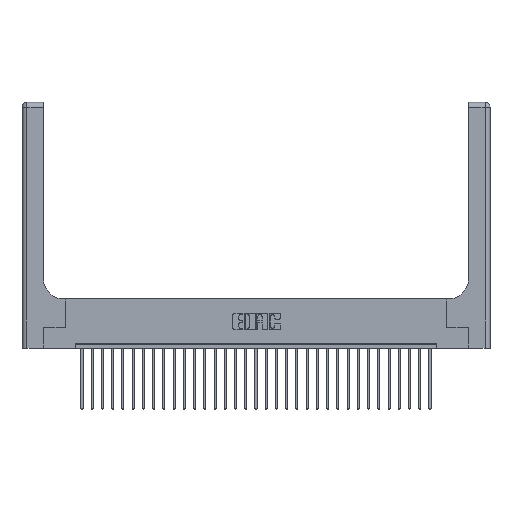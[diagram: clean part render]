
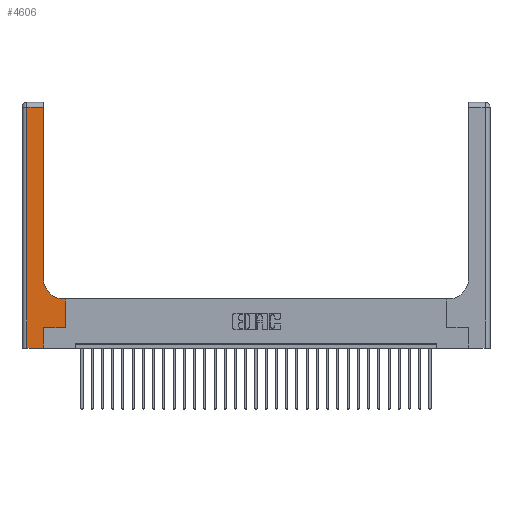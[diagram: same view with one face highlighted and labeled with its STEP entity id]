
A CAD part, top view. The second image highlights one B-rep face of the part: STEP entity #4606.
In plain terms, the highlighted planar face has unit normal (0, 0, 1).
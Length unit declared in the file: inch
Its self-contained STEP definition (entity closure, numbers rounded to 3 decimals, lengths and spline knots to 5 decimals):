
#72 = CARTESIAN_POINT ( 'NONE',  ( 0.26, 3., 0.37 ) ) ;
#588 = CARTESIAN_POINT ( 'NONE',  ( 0.265, 0.25, 0.37 ) ) ;
#1229 = CARTESIAN_POINT ( 'NONE',  ( 0., 0., 0.37 ) ) ;
#1297 = VECTOR ( 'NONE', #9552, 39.37008 ) ;
#1741 = LINE ( 'NONE', #25455, #25307 ) ;
#2475 = EDGE_CURVE ( 'NONE', #23902, #25149, #2634, .T. ) ;
#2634 = LINE ( 'NONE', #17850, #22500 ) ;
#3107 = CARTESIAN_POINT ( 'NONE',  ( 0.26, 2.94, 0.37 ) ) ;
#3252 = VERTEX_POINT ( 'NONE', #21655 ) ;
#3727 = AXIS2_PLACEMENT_3D ( 'NONE', #21616, #21528, #19169 ) ;
#3817 = CIRCLE ( 'NONE', #18134, 0.25 ) ;
#4252 = PLANE ( 'NONE',  #3727 ) ;
#4606 = ADVANCED_FACE ( 'NONE', ( #6534 ), #4252, .F. ) ;
#5567 = DIRECTION ( 'NONE',  ( 0., 0., -1. ) ) ;
#6486 = LINE ( 'NONE', #17492, #7158 ) ;
#6534 = FACE_OUTER_BOUND ( 'NONE', #21782, .T. ) ;
#6974 = LINE ( 'NONE', #14056, #1297 ) ;
#7095 = VERTEX_POINT ( 'NONE', #588 ) ;
#7158 = VECTOR ( 'NONE', #13905, 39.37008 ) ;
#7409 = ORIENTED_EDGE ( 'NONE', *, *, #11218, .T. ) ;
#7798 = DIRECTION ( 'NONE',  ( 1., 0., 0. ) ) ;
#9189 = DIRECTION ( 'NONE',  ( 1., 0., 0. ) ) ;
#9239 = EDGE_CURVE ( 'NONE', #14767, #23902, #10029, .T. ) ;
#9552 = DIRECTION ( 'NONE',  ( -1., 0., 0. ) ) ;
#9824 = CARTESIAN_POINT ( 'NONE',  ( 0.26, 0.85, 0.37 ) ) ;
#10029 = LINE ( 'NONE', #72, #26549 ) ;
#10254 = LINE ( 'NONE', #13310, #17614 ) ;
#10603 = LINE ( 'NONE', #22270, #11279 ) ;
#11218 = EDGE_CURVE ( 'NONE', #7095, #3252, #10254, .T. ) ;
#11279 = VECTOR ( 'NONE', #17810, 39.37008 ) ;
#11378 = EDGE_CURVE ( 'NONE', #23360, #19097, #16953, .T. ) ;
#13310 = CARTESIAN_POINT ( 'NONE',  ( 0.265, 0.25, 0.37 ) ) ;
#13905 = DIRECTION ( 'NONE',  ( 0., 1., 0. ) ) ;
#14056 = CARTESIAN_POINT ( 'NONE',  ( 0.26, 0.6, 0.37 ) ) ;
#14581 = CARTESIAN_POINT ( 'NONE',  ( 0.51, 0.6, 0.37 ) ) ;
#14767 = VERTEX_POINT ( 'NONE', #9824 ) ;
#14799 = VERTEX_POINT ( 'NONE', #21322 ) ;
#15050 = DIRECTION ( 'NONE',  ( 0., 1., 0. ) ) ;
#15445 = EDGE_CURVE ( 'NONE', #18345, #14767, #3817, .T. ) ;
#16411 = ORIENTED_EDGE ( 'NONE', *, *, #20145, .T. ) ;
#16953 = LINE ( 'NONE', #1229, #21362 ) ;
#17057 = CARTESIAN_POINT ( 'NONE',  ( 0.06, 2.94, 0.37 ) ) ;
#17492 = CARTESIAN_POINT ( 'NONE',  ( 0.528, 0.25, 0.37 ) ) ;
#17614 = VECTOR ( 'NONE', #9189, 39.37008 ) ;
#17810 = DIRECTION ( 'NONE',  ( 0., 1., 0. ) ) ;
#17850 = CARTESIAN_POINT ( 'NONE',  ( 0., 2.94, 0.37 ) ) ;
#18134 = AXIS2_PLACEMENT_3D ( 'NONE', #18416, #5567, #7798 ) ;
#18345 = VERTEX_POINT ( 'NONE', #14581 ) ;
#18416 = CARTESIAN_POINT ( 'NONE',  ( 0.51, 0.85, 0.37 ) ) ;
#18656 = DIRECTION ( 'NONE',  ( 0., -1., 0. ) ) ;
#18945 = ORIENTED_EDGE ( 'NONE', *, *, #9239, .T. ) ;
#19086 = ORIENTED_EDGE ( 'NONE', *, *, #15445, .T. ) ;
#19097 = VERTEX_POINT ( 'NONE', #26027 ) ;
#19169 = DIRECTION ( 'NONE',  ( -1., 0., 0. ) ) ;
#20145 = EDGE_CURVE ( 'NONE', #25149, #23360, #1741, .T. ) ;
#21290 = ORIENTED_EDGE ( 'NONE', *, *, #11378, .T. ) ;
#21322 = CARTESIAN_POINT ( 'NONE',  ( 0.528, 0.6, 0.37 ) ) ;
#21362 = VECTOR ( 'NONE', #24729, 39.37008 ) ;
#21528 = DIRECTION ( 'NONE',  ( 0., 0., -1. ) ) ;
#21616 = CARTESIAN_POINT ( 'NONE',  ( 0., 3., 0.37 ) ) ;
#21655 = CARTESIAN_POINT ( 'NONE',  ( 0.528, 0.25, 0.37 ) ) ;
#21782 = EDGE_LOOP ( 'NONE', ( #18945, #25290, #16411, #21290, #23550, #7409, #27173, #22607, #19086 ) ) ;
#21960 = EDGE_CURVE ( 'NONE', #14799, #18345, #6974, .T. ) ;
#22270 = CARTESIAN_POINT ( 'NONE',  ( 0.265, 0., 0.37 ) ) ;
#22329 = CARTESIAN_POINT ( 'NONE',  ( 0.06, 0., 0.37 ) ) ;
#22500 = VECTOR ( 'NONE', #24221, 39.37008 ) ;
#22607 = ORIENTED_EDGE ( 'NONE', *, *, #21960, .T. ) ;
#23360 = VERTEX_POINT ( 'NONE', #22329 ) ;
#23550 = ORIENTED_EDGE ( 'NONE', *, *, #26607, .T. ) ;
#23902 = VERTEX_POINT ( 'NONE', #3107 ) ;
#24221 = DIRECTION ( 'NONE',  ( -1., 0., 0. ) ) ;
#24729 = DIRECTION ( 'NONE',  ( 1., 0., 0. ) ) ;
#25149 = VERTEX_POINT ( 'NONE', #17057 ) ;
#25290 = ORIENTED_EDGE ( 'NONE', *, *, #2475, .T. ) ;
#25307 = VECTOR ( 'NONE', #18656, 39.37008 ) ;
#25455 = CARTESIAN_POINT ( 'NONE',  ( 0.06, 3., 0.37 ) ) ;
#25519 = EDGE_CURVE ( 'NONE', #3252, #14799, #6486, .T. ) ;
#26027 = CARTESIAN_POINT ( 'NONE',  ( 0.265, 0., 0.37 ) ) ;
#26549 = VECTOR ( 'NONE', #15050, 39.37008 ) ;
#26607 = EDGE_CURVE ( 'NONE', #19097, #7095, #10603, .T. ) ;
#27173 = ORIENTED_EDGE ( 'NONE', *, *, #25519, .T. ) ;
